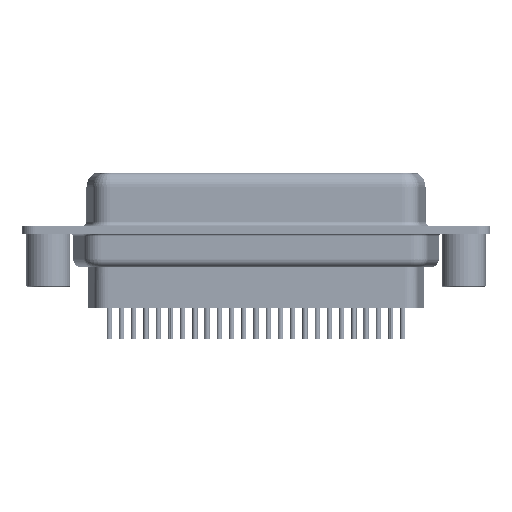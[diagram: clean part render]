
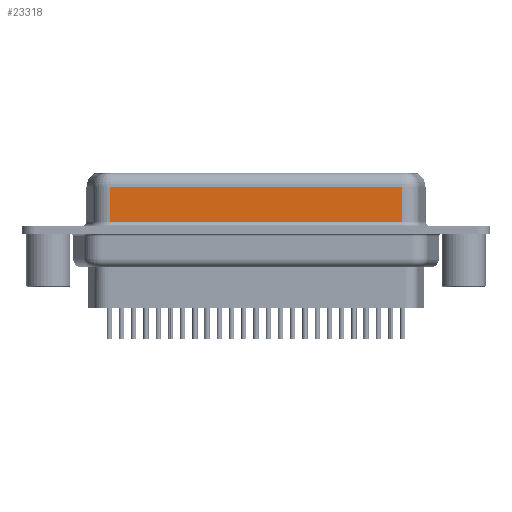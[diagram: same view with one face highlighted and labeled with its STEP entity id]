
A CAD part, front view. The second image highlights one B-rep face of the part: STEP entity #23318.
In plain terms, the highlighted planar face has unit normal (0, -1, 0).
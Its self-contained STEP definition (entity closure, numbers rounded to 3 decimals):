
#17 = ORIENTED_EDGE ( 'NONE', *, *, #11387, .T. ) ;
#1440 = AXIS2_PLACEMENT_3D ( 'NONE', #2733, #16624, #30635 ) ;
#2127 = PLANE ( 'NONE',  #1440 ) ;
#2168 = LINE ( 'NONE', #25696, #29620 ) ;
#2733 = CARTESIAN_POINT ( 'NONE',  ( 40.032, -3.95, 6.6 ) ) ;
#2805 = DIRECTION ( 'NONE',  ( 1., 0., 0. ) ) ;
#2946 = CARTESIAN_POINT ( 'NONE',  ( 40.032, -3.95, 0.95 ) ) ;
#4151 = VECTOR ( 'NONE', #24322, 1000. ) ;
#4167 = DIRECTION ( 'NONE',  ( 0., 0., -1. ) ) ;
#4441 = VERTEX_POINT ( 'NONE', #14098 ) ;
#5592 = VERTEX_POINT ( 'NONE', #2946 ) ;
#6870 = VECTOR ( 'NONE', #2805, 1000. ) ;
#7331 = LINE ( 'NONE', #26345, #4151 ) ;
#10287 = EDGE_LOOP ( 'NONE', ( #12326, #17, #26706, #13412 ) ) ;
#11182 = CARTESIAN_POINT ( 'NONE',  ( 40.032, -3.95, 6.6 ) ) ;
#11387 = EDGE_CURVE ( 'NONE', #29202, #14495, #2168, .T. ) ;
#12019 = CARTESIAN_POINT ( 'NONE',  ( 40.032, -3.95, 0.95 ) ) ;
#12326 = ORIENTED_EDGE ( 'NONE', *, *, #26073, .F. ) ;
#13412 = ORIENTED_EDGE ( 'NONE', *, *, #22416, .T. ) ;
#14098 = CARTESIAN_POINT ( 'NONE',  ( 7.008, -3.95, 0.95 ) ) ;
#14495 = VERTEX_POINT ( 'NONE', #23097 ) ;
#16021 = EDGE_CURVE ( 'NONE', #14495, #4441, #7331, .T. ) ;
#16624 = DIRECTION ( 'NONE',  ( 0., 1., 0. ) ) ;
#18221 = DIRECTION ( 'NONE',  ( -1., 0., 0. ) ) ;
#19831 = VECTOR ( 'NONE', #4167, 1000. ) ;
#22416 = EDGE_CURVE ( 'NONE', #4441, #5592, #28669, .T. ) ;
#23097 = CARTESIAN_POINT ( 'NONE',  ( 7.008, -3.95, 4.85 ) ) ;
#23318 = ADVANCED_FACE ( 'NONE', ( #25810 ), #2127, .F. ) ;
#24322 = DIRECTION ( 'NONE',  ( 0., 0., -1. ) ) ;
#25696 = CARTESIAN_POINT ( 'NONE',  ( 40.032, -3.95, 4.85 ) ) ;
#25810 = FACE_OUTER_BOUND ( 'NONE', #10287, .T. ) ;
#26073 = EDGE_CURVE ( 'NONE', #29202, #5592, #30491, .T. ) ;
#26345 = CARTESIAN_POINT ( 'NONE',  ( 7.008, -3.95, 6.6 ) ) ;
#26706 = ORIENTED_EDGE ( 'NONE', *, *, #16021, .T. ) ;
#27056 = CARTESIAN_POINT ( 'NONE',  ( 40.032, -3.95, 4.85 ) ) ;
#28669 = LINE ( 'NONE', #12019, #6870 ) ;
#29202 = VERTEX_POINT ( 'NONE', #27056 ) ;
#29620 = VECTOR ( 'NONE', #18221, 1000. ) ;
#30491 = LINE ( 'NONE', #11182, #19831 ) ;
#30635 = DIRECTION ( 'NONE',  ( 0., 0., 1. ) ) ;
